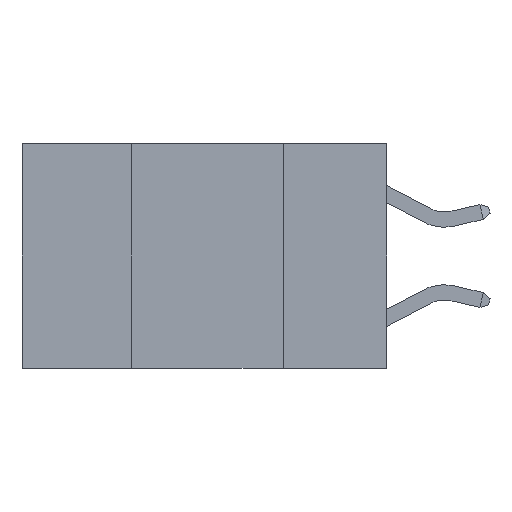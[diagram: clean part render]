
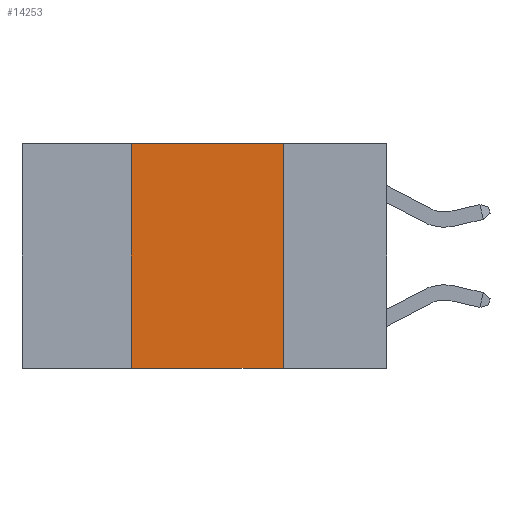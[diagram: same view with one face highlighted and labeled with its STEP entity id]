
A CAD part, left-side view. The second image highlights one B-rep face of the part: STEP entity #14253.
In plain terms, the highlighted planar face has unit normal (-1, 0, 0).
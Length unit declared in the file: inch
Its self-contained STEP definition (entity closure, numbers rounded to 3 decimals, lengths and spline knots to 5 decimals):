
#522 = CARTESIAN_POINT ( 'NONE',  ( 0., 0.42, 0. ) ) ;
#1056 = LINE ( 'NONE', #5974, #4258 ) ;
#1290 = EDGE_CURVE ( 'NONE', #7640, #5459, #1056, .T. ) ;
#1613 = DIRECTION ( 'NONE',  ( 1., 0., 0. ) ) ;
#1897 = ORIENTED_EDGE ( 'NONE', *, *, #3716, .F. ) ;
#2831 = VECTOR ( 'NONE', #5600, 39.37008 ) ;
#3126 = DIRECTION ( 'NONE',  ( 0., -1., 0. ) ) ;
#3716 = EDGE_CURVE ( 'NONE', #14209, #5610, #15197, .T. ) ;
#4031 = CARTESIAN_POINT ( 'NONE',  ( 0., 0.6, -0.37 ) ) ;
#4258 = VECTOR ( 'NONE', #5901, 39.37008 ) ;
#4865 = LINE ( 'NONE', #9787, #8750 ) ;
#5194 = EDGE_LOOP ( 'NONE', ( #8728, #15467, #1897, #8388 ) ) ;
#5436 = EDGE_CURVE ( 'NONE', #5610, #7640, #4865, .T. ) ;
#5459 = VERTEX_POINT ( 'NONE', #7214 ) ;
#5600 = DIRECTION ( 'NONE',  ( 0., 0., 1. ) ) ;
#5610 = VERTEX_POINT ( 'NONE', #7901 ) ;
#5901 = DIRECTION ( 'NONE',  ( 0., 0., -1. ) ) ;
#5974 = CARTESIAN_POINT ( 'NONE',  ( 0., 0.17, 0. ) ) ;
#7014 = VECTOR ( 'NONE', #3126, 39.37008 ) ;
#7214 = CARTESIAN_POINT ( 'NONE',  ( 0., 0.17, -0.37 ) ) ;
#7640 = VERTEX_POINT ( 'NONE', #10750 ) ;
#7750 = FACE_OUTER_BOUND ( 'NONE', #5194, .T. ) ;
#7901 = CARTESIAN_POINT ( 'NONE',  ( 0., 0.42, 0. ) ) ;
#8388 = ORIENTED_EDGE ( 'NONE', *, *, #8778, .T. ) ;
#8728 = ORIENTED_EDGE ( 'NONE', *, *, #1290, .F. ) ;
#8750 = VECTOR ( 'NONE', #13209, 39.37008 ) ;
#8778 = EDGE_CURVE ( 'NONE', #14209, #5459, #9265, .T. ) ;
#9265 = LINE ( 'NONE', #4031, #7014 ) ;
#9787 = CARTESIAN_POINT ( 'NONE',  ( 0., 0.6, 0. ) ) ;
#10205 = AXIS2_PLACEMENT_3D ( 'NONE', #10240, #1613, #11265 ) ;
#10240 = CARTESIAN_POINT ( 'NONE',  ( 0., 0.6, 0. ) ) ;
#10750 = CARTESIAN_POINT ( 'NONE',  ( 0., 0.17, 0. ) ) ;
#11265 = DIRECTION ( 'NONE',  ( 0., 0., -1. ) ) ;
#11432 = CARTESIAN_POINT ( 'NONE',  ( 0., 0.42, -0.37 ) ) ;
#12627 = PLANE ( 'NONE',  #10205 ) ;
#13209 = DIRECTION ( 'NONE',  ( 0., -1., 0. ) ) ;
#14209 = VERTEX_POINT ( 'NONE', #11432 ) ;
#14253 = ADVANCED_FACE ( 'NONE', ( #7750 ), #12627, .F. ) ;
#15197 = LINE ( 'NONE', #522, #2831 ) ;
#15467 = ORIENTED_EDGE ( 'NONE', *, *, #5436, .F. ) ;
